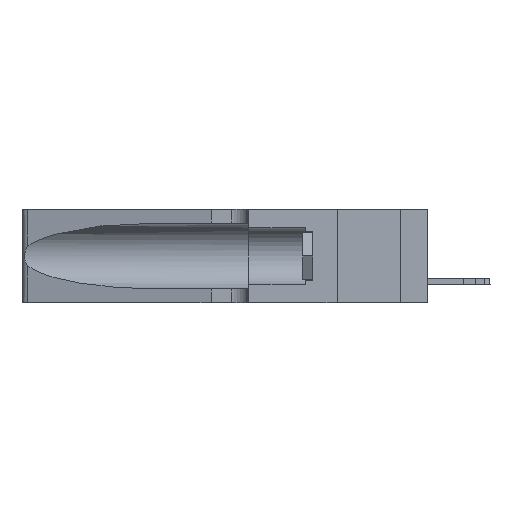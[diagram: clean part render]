
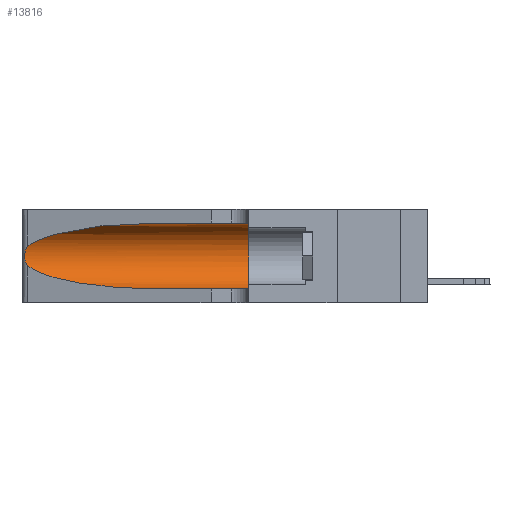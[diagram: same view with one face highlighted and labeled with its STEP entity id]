
A CAD part, left-side view. The second image highlights one B-rep face of the part: STEP entity #13816.
In plain terms, the highlighted cylindrical face has radius 3.308 mm (diameter 6.617 mm), a partial arc.
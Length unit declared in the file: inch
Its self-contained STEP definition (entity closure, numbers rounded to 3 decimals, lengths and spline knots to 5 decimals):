
#177 = CARTESIAN_POINT ( 'NONE',  ( 0.18966, 0.96281, 0.05475 ) ) ;
#423 = CARTESIAN_POINT ( 'NONE',  ( 0.1305, 0.72297, 0.05475 ) ) ;
#672 = CARTESIAN_POINT ( 'NONE',  ( 0.26017, 1.23833, 0.17102 ) ) ;
#776 = AXIS2_PLACEMENT_3D ( 'NONE', #20132, #10863, #16773 ) ;
#1255 = DIRECTION ( 'NONE',  ( 0., 0., 1. ) ) ;
#1835 = CARTESIAN_POINT ( 'NONE',  ( 0.1305, 0.72297, 0.31525 ) ) ;
#2161 = CARTESIAN_POINT ( 'NONE',  ( 0.2373, 1.15595, 0.28018 ) ) ;
#2239 = ORIENTED_EDGE ( 'NONE', *, *, #37049, .T. ) ;
#5023 = CARTESIAN_POINT ( 'NONE',  ( 0.25487, 1.22718, 0.22369 ) ) ;
#5025 = ORIENTED_EDGE ( 'NONE', *, *, #15628, .F. ) ;
#6823 = EDGE_CURVE ( 'NONE', #31136, #13646, #18435, .T. ) ;
#6849 = FACE_OUTER_BOUND ( 'NONE', #9772, .T. ) ;
#8900 = CARTESIAN_POINT ( 'NONE',  ( 0.1305, 0.35, 0.185 ) ) ;
#9088 = CARTESIAN_POINT ( 'NONE',  ( 0.25787, 1.23484, 0.2124 ) ) ;
#9772 = EDGE_LOOP ( 'NONE', ( #29332, #13980, #23456, #2239, #20249, #5025 ) ) ;
#10696 = CARTESIAN_POINT ( 'NONE',  ( 0.1305, 0.72297, 0.31525 ) ) ;
#10863 = DIRECTION ( 'NONE',  ( 0., -1., 0. ) ) ;
#11928 = CARTESIAN_POINT ( 'NONE',  ( 0.25789, 1.23486, 0.15765 ) ) ;
#12425 = CARTESIAN_POINT ( 'NONE',  ( 0.25854, 1.2359, 0.20912 ) ) ;
#12702 = LINE ( 'NONE', #35007, #34794 ) ;
#13646 = VERTEX_POINT ( 'NONE', #28580 ) ;
#13816 = ADVANCED_FACE ( 'NONE', ( #6849 ), #36316, .F. ) ;
#13980 = ORIENTED_EDGE ( 'NONE', *, *, #33637, .T. ) ;
#15152 = CARTESIAN_POINT ( 'NONE',  ( 0.25487, 1.22718, 0.14631 ) ) ;
#15395 = CARTESIAN_POINT ( 'NONE',  ( 0.26075, 1.23896, 0.178 ) ) ;
#15628 = EDGE_CURVE ( 'NONE', #17589, #31136, #12702, .T. ) ;
#16609 = CARTESIAN_POINT ( 'NONE',  ( 0.18966, 0.96281, 0.31525 ) ) ;
#16773 = DIRECTION ( 'NONE',  ( 0., 0., -1. ) ) ;
#17589 = VERTEX_POINT ( 'NONE', #1835 ) ;
#18253 = CARTESIAN_POINT ( 'NONE',  ( 0.1305, 0.72297, 0.05475 ) ) ;
#18268 = VERTEX_POINT ( 'NONE', #18253 ) ;
#18435 = CIRCLE ( 'NONE', #37196, 0.13025 ) ;
#18752 = LINE ( 'NONE', #26784, #21547 ) ;
#19795 = VERTEX_POINT ( 'NONE', #29795 ) ;
#20132 = CARTESIAN_POINT ( 'NONE',  ( 0.1305, 1.61858, 0.185 ) ) ;
#20221 = DIRECTION ( 'NONE',  ( 0., -1., 0. ) ) ;
#20249 = ORIENTED_EDGE ( 'NONE', *, *, #6823, .F. ) ;
#21067 = CARTESIAN_POINT ( 'NONE',  ( 0.25487, 1.22718, 0.22369 ) ) ;
#21547 = VECTOR ( 'NONE', #35456, 39.37008 ) ;
#21686 = B_SPLINE_CURVE_WITH_KNOTS ( 'NONE', 3,
 ( #21067, #27164, #30112, #9088, #12425, #33007, #26792, #15395, #672, #24355, #11928, #32525, #35589, #15152 ),
 .UNSPECIFIED., .F., .F.,
 ( 4, 2, 2, 2, 2, 2, 4 ),
 ( 0., 0.00027, 0.00053, 0.00107, 0.0016, 0.00187, 0.00214 ),
 .UNSPECIFIED. ) ;
#23456 = ORIENTED_EDGE ( 'NONE', *, *, #30837, .T. ) ;
#23621 = EDGE_CURVE ( 'NONE', #17589, #27803, #26228, .T. ) ;
#24355 = CARTESIAN_POINT ( 'NONE',  ( 0.25856, 1.23593, 0.16098 ) ) ;
#25011 = DIRECTION ( 'NONE',  ( 0., 1., 0. ) ) ;
#25930 = CARTESIAN_POINT ( 'NONE',  ( 0.2373, 1.15595, 0.08982 ) ) ;
#26228 =( BOUNDED_CURVE ( )  B_SPLINE_CURVE ( 3, ( #10696, #16609, #2161, #5023 ),
 .UNSPECIFIED., .F., .T. ) 
 B_SPLINE_CURVE_WITH_KNOTS ( ( 4, 4 ),
 ( 1.5708, 2.84003 ),
 .UNSPECIFIED. ) 
 CURVE ( )  GEOMETRIC_REPRESENTATION_ITEM ( )  RATIONAL_B_SPLINE_CURVE ( ( 1., 0.87, 0.87, 1. ) ) 
 REPRESENTATION_ITEM ( '' )  );
#26784 = CARTESIAN_POINT ( 'NONE',  ( 0.1305, 1.61858, 0.05475 ) ) ;
#26792 = CARTESIAN_POINT ( 'NONE',  ( 0.26075, 1.23896, 0.19203 ) ) ;
#27164 = CARTESIAN_POINT ( 'NONE',  ( 0.25555, 1.22994, 0.2215 ) ) ;
#27803 = VERTEX_POINT ( 'NONE', #36006 ) ;
#28566 =( BOUNDED_CURVE ( )  B_SPLINE_CURVE ( 3, ( #37963, #25930, #177, #423 ),
 .UNSPECIFIED., .F., .T. ) 
 B_SPLINE_CURVE_WITH_KNOTS ( ( 4, 4 ),
 ( 3.44316, 4.71239 ),
 .UNSPECIFIED. ) 
 CURVE ( )  GEOMETRIC_REPRESENTATION_ITEM ( )  RATIONAL_B_SPLINE_CURVE ( ( 1., 0.87, 0.87, 1. ) ) 
 REPRESENTATION_ITEM ( '' )  );
#28580 = CARTESIAN_POINT ( 'NONE',  ( 0.1305, 0.35, 0.05475 ) ) ;
#29332 = ORIENTED_EDGE ( 'NONE', *, *, #23621, .T. ) ;
#29795 = CARTESIAN_POINT ( 'NONE',  ( 0.25487, 1.22718, 0.14631 ) ) ;
#29838 = CARTESIAN_POINT ( 'NONE',  ( 0.1305, 0.35, 0.31525 ) ) ;
#30112 = CARTESIAN_POINT ( 'NONE',  ( 0.25639, 1.23184, 0.21858 ) ) ;
#30837 = EDGE_CURVE ( 'NONE', #19795, #18268, #28566, .T. ) ;
#31136 = VERTEX_POINT ( 'NONE', #29838 ) ;
#32525 = CARTESIAN_POINT ( 'NONE',  ( 0.25639, 1.23186, 0.15144 ) ) ;
#33007 = CARTESIAN_POINT ( 'NONE',  ( 0.26018, 1.23835, 0.19895 ) ) ;
#33637 = EDGE_CURVE ( 'NONE', #27803, #19795, #21686, .T. ) ;
#34794 = VECTOR ( 'NONE', #20221, 39.37008 ) ;
#35007 = CARTESIAN_POINT ( 'NONE',  ( 0.1305, 1.61858, 0.31525 ) ) ;
#35456 = DIRECTION ( 'NONE',  ( 0., -1., 0. ) ) ;
#35589 = CARTESIAN_POINT ( 'NONE',  ( 0.25555, 1.22993, 0.14849 ) ) ;
#36006 = CARTESIAN_POINT ( 'NONE',  ( 0.25487, 1.22718, 0.22369 ) ) ;
#36316 = CYLINDRICAL_SURFACE ( 'NONE', #776, 0.13025 ) ;
#37049 = EDGE_CURVE ( 'NONE', #18268, #13646, #18752, .T. ) ;
#37196 = AXIS2_PLACEMENT_3D ( 'NONE', #8900, #25011, #1255 ) ;
#37963 = CARTESIAN_POINT ( 'NONE',  ( 0.25487, 1.22718, 0.14631 ) ) ;
